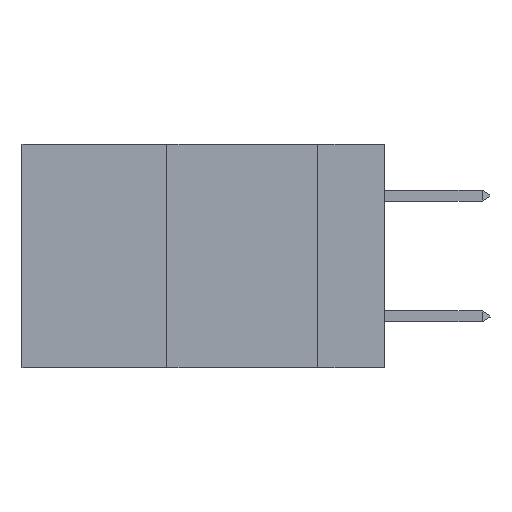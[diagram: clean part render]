
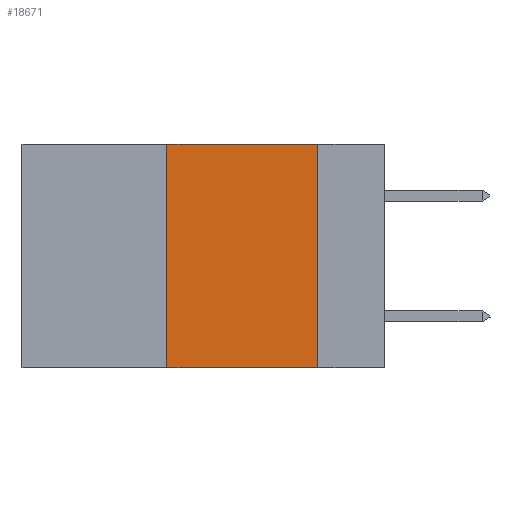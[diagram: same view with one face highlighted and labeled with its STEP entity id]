
A CAD part, left-side view. The second image highlights one B-rep face of the part: STEP entity #18671.
In plain terms, the highlighted planar face has unit normal (-1, 0, 0).
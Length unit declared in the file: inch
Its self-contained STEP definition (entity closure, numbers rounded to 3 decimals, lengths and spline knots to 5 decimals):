
#407 = VECTOR ( 'NONE', #26218, 39.37008 ) ;
#1844 = VECTOR ( 'NONE', #11079, 39.37008 ) ;
#1926 = AXIS2_PLACEMENT_3D ( 'NONE', #5064, #6975, #19000 ) ;
#3196 = FACE_OUTER_BOUND ( 'NONE', #21801, .T. ) ;
#4039 = LINE ( 'NONE', #11876, #7069 ) ;
#5064 = CARTESIAN_POINT ( 'NONE',  ( 0., 0.6, 0. ) ) ;
#5666 = LINE ( 'NONE', #18101, #7903 ) ;
#6975 = DIRECTION ( 'NONE',  ( 1., 0., 0. ) ) ;
#7069 = VECTOR ( 'NONE', #19869, 39.37008 ) ;
#7186 = CARTESIAN_POINT ( 'NONE',  ( 0., 0.11, 0. ) ) ;
#7340 = EDGE_CURVE ( 'NONE', #11961, #11140, #4039, .T. ) ;
#7903 = VECTOR ( 'NONE', #26152, 39.37008 ) ;
#7955 = CARTESIAN_POINT ( 'NONE',  ( 0., 0.11, 0. ) ) ;
#7980 = CARTESIAN_POINT ( 'NONE',  ( 0., 0.36, -0.37 ) ) ;
#8644 = CARTESIAN_POINT ( 'NONE',  ( 0., 0.36, 0. ) ) ;
#8907 = EDGE_CURVE ( 'NONE', #14697, #11140, #25527, .T. ) ;
#9583 = ORIENTED_EDGE ( 'NONE', *, *, #15984, .F. ) ;
#11079 = DIRECTION ( 'NONE',  ( 0., 0., -1. ) ) ;
#11140 = VERTEX_POINT ( 'NONE', #25294 ) ;
#11876 = CARTESIAN_POINT ( 'NONE',  ( 0., 0.6, -0.37 ) ) ;
#11961 = VERTEX_POINT ( 'NONE', #7980 ) ;
#13341 = ORIENTED_EDGE ( 'NONE', *, *, #26195, .F. ) ;
#14697 = VERTEX_POINT ( 'NONE', #7955 ) ;
#14948 = LINE ( 'NONE', #8644, #407 ) ;
#15984 = EDGE_CURVE ( 'NONE', #24712, #14697, #5666, .T. ) ;
#17163 = ORIENTED_EDGE ( 'NONE', *, *, #7340, .T. ) ;
#18101 = CARTESIAN_POINT ( 'NONE',  ( 0., 0.6, 0. ) ) ;
#18671 = ADVANCED_FACE ( 'NONE', ( #3196 ), #23418, .F. ) ;
#19000 = DIRECTION ( 'NONE',  ( 0., 0., -1. ) ) ;
#19869 = DIRECTION ( 'NONE',  ( 0., -1., 0. ) ) ;
#21801 = EDGE_LOOP ( 'NONE', ( #22296, #9583, #13341, #17163 ) ) ;
#22296 = ORIENTED_EDGE ( 'NONE', *, *, #8907, .F. ) ;
#23418 = PLANE ( 'NONE',  #1926 ) ;
#24712 = VERTEX_POINT ( 'NONE', #25808 ) ;
#25294 = CARTESIAN_POINT ( 'NONE',  ( 0., 0.11, -0.37 ) ) ;
#25527 = LINE ( 'NONE', #7186, #1844 ) ;
#25808 = CARTESIAN_POINT ( 'NONE',  ( 0., 0.36, 0. ) ) ;
#26152 = DIRECTION ( 'NONE',  ( 0., -1., 0. ) ) ;
#26195 = EDGE_CURVE ( 'NONE', #11961, #24712, #14948, .T. ) ;
#26218 = DIRECTION ( 'NONE',  ( 0., 0., 1. ) ) ;
